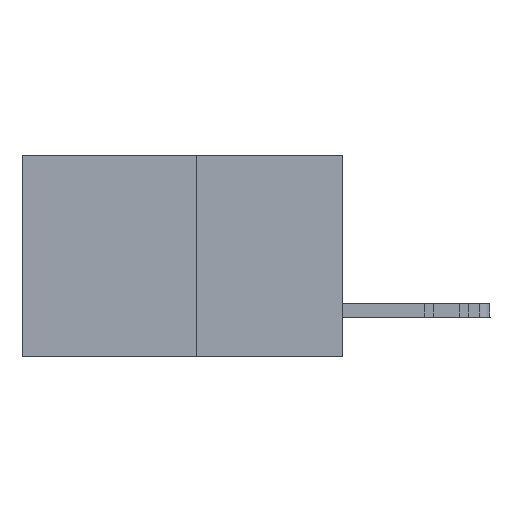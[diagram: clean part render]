
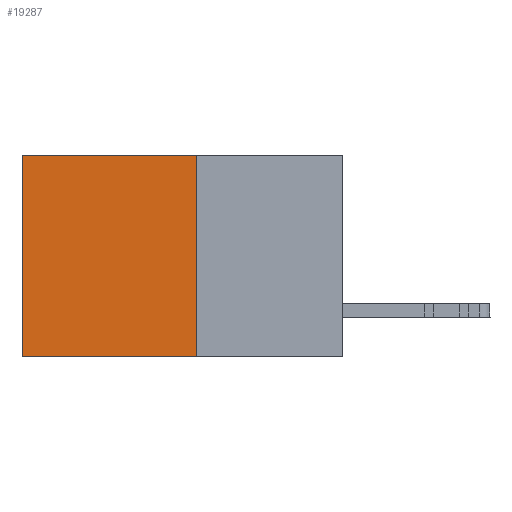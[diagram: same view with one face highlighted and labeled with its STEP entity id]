
A CAD part, left-side view. The second image highlights one B-rep face of the part: STEP entity #19287.
In plain terms, the highlighted planar face has unit normal (-1, 0, 0).
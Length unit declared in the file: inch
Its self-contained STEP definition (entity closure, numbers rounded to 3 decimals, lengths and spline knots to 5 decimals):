
#773 = DIRECTION ( 'NONE',  ( 0., 1., 0. ) ) ;
#1412 = EDGE_LOOP ( 'NONE', ( #5539, #3173, #12840, #14026 ) ) ;
#2446 = CARTESIAN_POINT ( 'NONE',  ( 0.277, 0.27, -0.37 ) ) ;
#2466 = VERTEX_POINT ( 'NONE', #32374 ) ;
#3173 = ORIENTED_EDGE ( 'NONE', *, *, #23268, .F. ) ;
#3671 = CARTESIAN_POINT ( 'NONE',  ( 0.277, 0.59, 0. ) ) ;
#4126 = LINE ( 'NONE', #10794, #30152 ) ;
#5539 = ORIENTED_EDGE ( 'NONE', *, *, #16449, .T. ) ;
#6672 = LINE ( 'NONE', #16049, #32717 ) ;
#6804 = VERTEX_POINT ( 'NONE', #10193 ) ;
#7503 = DIRECTION ( 'NONE',  ( 0., 0., -1. ) ) ;
#7893 = EDGE_CURVE ( 'NONE', #9705, #2466, #32557, .T. ) ;
#8132 = AXIS2_PLACEMENT_3D ( 'NONE', #2446, #22618, #7503 ) ;
#9705 = VERTEX_POINT ( 'NONE', #27676 ) ;
#10193 = CARTESIAN_POINT ( 'NONE',  ( 0.277, 0.59, -0.37 ) ) ;
#10624 = EDGE_CURVE ( 'NONE', #9705, #21468, #4126, .T. ) ;
#10794 = CARTESIAN_POINT ( 'NONE',  ( 0.277, 0.27, 0. ) ) ;
#11074 = LINE ( 'NONE', #32224, #17777 ) ;
#12459 = FACE_OUTER_BOUND ( 'NONE', #1412, .T. ) ;
#12840 = ORIENTED_EDGE ( 'NONE', *, *, #7893, .F. ) ;
#14026 = ORIENTED_EDGE ( 'NONE', *, *, #10624, .T. ) ;
#14236 = CARTESIAN_POINT ( 'NONE',  ( 0.277, 0.27, -0.37 ) ) ;
#14994 = PLANE ( 'NONE',  #8132 ) ;
#16049 = CARTESIAN_POINT ( 'NONE',  ( 0.277, 0.59, -0.37 ) ) ;
#16449 = EDGE_CURVE ( 'NONE', #21468, #6804, #6672, .T. ) ;
#17777 = VECTOR ( 'NONE', #22199, 39.37008 ) ;
#19287 = ADVANCED_FACE ( 'NONE', ( #12459 ), #14994, .F. ) ;
#21468 = VERTEX_POINT ( 'NONE', #3671 ) ;
#21846 = DIRECTION ( 'NONE',  ( 0., 0., -1. ) ) ;
#22199 = DIRECTION ( 'NONE',  ( 0., 1., 0. ) ) ;
#22618 = DIRECTION ( 'NONE',  ( 1., 0., 0. ) ) ;
#23268 = EDGE_CURVE ( 'NONE', #2466, #6804, #11074, .T. ) ;
#25086 = VECTOR ( 'NONE', #21846, 39.37008 ) ;
#27676 = CARTESIAN_POINT ( 'NONE',  ( 0.277, 0.27, 0. ) ) ;
#30152 = VECTOR ( 'NONE', #773, 39.37008 ) ;
#31194 = DIRECTION ( 'NONE',  ( 0., 0., -1. ) ) ;
#32224 = CARTESIAN_POINT ( 'NONE',  ( 0.277, 0.27, -0.37 ) ) ;
#32374 = CARTESIAN_POINT ( 'NONE',  ( 0.277, 0.27, -0.37 ) ) ;
#32557 = LINE ( 'NONE', #14236, #25086 ) ;
#32717 = VECTOR ( 'NONE', #31194, 39.37008 ) ;
